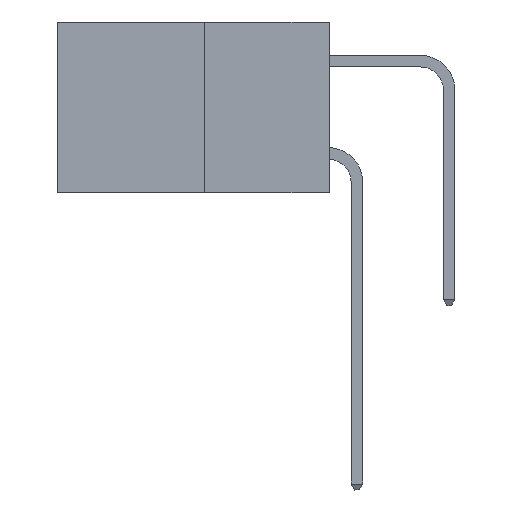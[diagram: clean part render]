
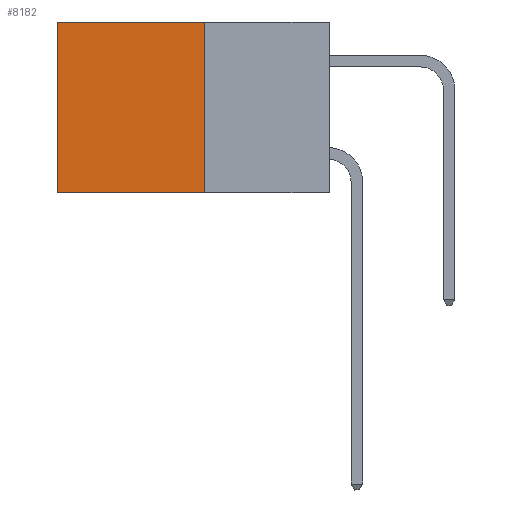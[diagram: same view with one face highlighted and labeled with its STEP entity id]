
A CAD part, left-side view. The second image highlights one B-rep face of the part: STEP entity #8182.
In plain terms, the highlighted planar face has unit normal (-1, 0, 0).
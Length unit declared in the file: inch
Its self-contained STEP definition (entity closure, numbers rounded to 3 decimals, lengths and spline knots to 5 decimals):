
#92 = ORIENTED_EDGE ( 'NONE', *, *, #195, .F. ) ;
#195 = EDGE_CURVE ( 'NONE', #16934, #22512, #15973, .T. ) ;
#265 = VECTOR ( 'NONE', #19541, 39.37008 ) ;
#404 = EDGE_CURVE ( 'NONE', #22512, #17306, #6740, .T. ) ;
#1110 = VECTOR ( 'NONE', #4455, 39.37008 ) ;
#2984 = CARTESIAN_POINT ( 'NONE',  ( 0.277, 0.59, -0.37 ) ) ;
#3984 = LINE ( 'NONE', #2984, #12669 ) ;
#4376 = CARTESIAN_POINT ( 'NONE',  ( 0.277, 0.59, 0. ) ) ;
#4455 = DIRECTION ( 'NONE',  ( 0., 0., -1. ) ) ;
#5279 = LINE ( 'NONE', #8438, #265 ) ;
#6199 = CARTESIAN_POINT ( 'NONE',  ( 0.277, 0.27, -0.37 ) ) ;
#6384 = ORIENTED_EDGE ( 'NONE', *, *, #12300, .T. ) ;
#6471 = FACE_OUTER_BOUND ( 'NONE', #20464, .T. ) ;
#6740 = LINE ( 'NONE', #12072, #20958 ) ;
#7710 = CARTESIAN_POINT ( 'NONE',  ( 0.277, 0.59, -0.37 ) ) ;
#8182 = ADVANCED_FACE ( 'NONE', ( #6471 ), #19974, .F. ) ;
#8438 = CARTESIAN_POINT ( 'NONE',  ( 0.277, 0.27, 0. ) ) ;
#12072 = CARTESIAN_POINT ( 'NONE',  ( 0.277, 0.27, -0.37 ) ) ;
#12205 = DIRECTION ( 'NONE',  ( 0., 0., -1. ) ) ;
#12274 = ORIENTED_EDGE ( 'NONE', *, *, #18811, .T. ) ;
#12300 = EDGE_CURVE ( 'NONE', #23787, #17306, #3984, .T. ) ;
#12669 = VECTOR ( 'NONE', #12205, 39.37008 ) ;
#15640 = CARTESIAN_POINT ( 'NONE',  ( 0.277, 0.27, -0.37 ) ) ;
#15857 = CARTESIAN_POINT ( 'NONE',  ( 0.277, 0.27, 0. ) ) ;
#15973 = LINE ( 'NONE', #15640, #1110 ) ;
#16803 = ORIENTED_EDGE ( 'NONE', *, *, #404, .F. ) ;
#16934 = VERTEX_POINT ( 'NONE', #15857 ) ;
#17306 = VERTEX_POINT ( 'NONE', #7710 ) ;
#18811 = EDGE_CURVE ( 'NONE', #16934, #23787, #5279, .T. ) ;
#19541 = DIRECTION ( 'NONE',  ( 0., 1., 0. ) ) ;
#19931 = DIRECTION ( 'NONE',  ( 0., 0., -1. ) ) ;
#19945 = DIRECTION ( 'NONE',  ( 1., 0., 0. ) ) ;
#19974 = PLANE ( 'NONE',  #23582 ) ;
#20033 = CARTESIAN_POINT ( 'NONE',  ( 0.277, 0.27, -0.37 ) ) ;
#20464 = EDGE_LOOP ( 'NONE', ( #6384, #16803, #92, #12274 ) ) ;
#20958 = VECTOR ( 'NONE', #23504, 39.37008 ) ;
#22512 = VERTEX_POINT ( 'NONE', #6199 ) ;
#23504 = DIRECTION ( 'NONE',  ( 0., 1., 0. ) ) ;
#23582 = AXIS2_PLACEMENT_3D ( 'NONE', #20033, #19945, #19931 ) ;
#23787 = VERTEX_POINT ( 'NONE', #4376 ) ;
